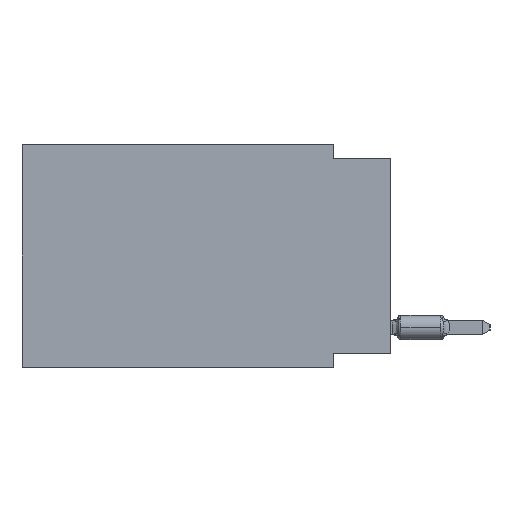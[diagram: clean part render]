
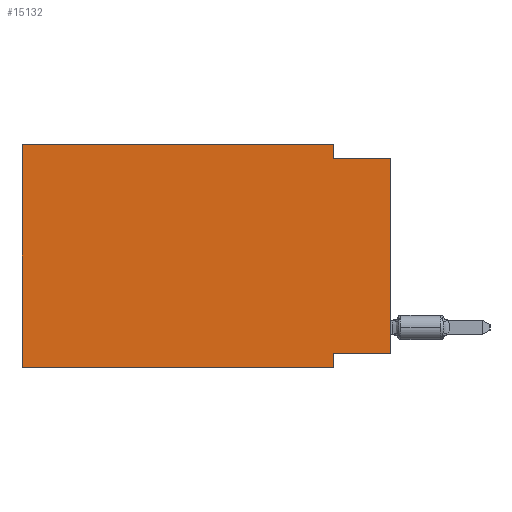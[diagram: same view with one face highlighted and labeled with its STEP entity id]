
A CAD part, left-side view. The second image highlights one B-rep face of the part: STEP entity #15132.
In plain terms, the highlighted planar face has unit normal (-1, 0, 0).
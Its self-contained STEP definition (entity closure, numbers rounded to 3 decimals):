
#46 = EDGE_CURVE ( 'NONE', #6103, #14184, #15102, .T. ) ;
#79 = CARTESIAN_POINT ( 'NONE',  ( 0., 16.383, -9.906 ) ) ;
#693 = ORIENTED_EDGE ( 'NONE', *, *, #7717, .T. ) ;
#972 = PLANE ( 'NONE',  #1155 ) ;
#1155 = AXIS2_PLACEMENT_3D ( 'NONE', #4593, #9602, #20739 ) ;
#1368 = EDGE_CURVE ( 'NONE', #10197, #13749, #8727, .T. ) ;
#1797 = ORIENTED_EDGE ( 'NONE', *, *, #46, .F. ) ;
#1824 = VECTOR ( 'NONE', #12740, 1000. ) ;
#1884 = CARTESIAN_POINT ( 'NONE',  ( 0., 2.54, 0. ) ) ;
#2053 = ORIENTED_EDGE ( 'NONE', *, *, #5603, .F. ) ;
#2114 = CARTESIAN_POINT ( 'NONE',  ( 0., 0., 0. ) ) ;
#2414 = VECTOR ( 'NONE', #20192, 1000. ) ;
#2853 = LINE ( 'NONE', #16040, #5142 ) ;
#2958 = CARTESIAN_POINT ( 'NONE',  ( 0., 2.54, -9.906 ) ) ;
#4232 = VECTOR ( 'NONE', #5402, 1000. ) ;
#4593 = CARTESIAN_POINT ( 'NONE',  ( 0., 16.383, 0. ) ) ;
#5037 = ORIENTED_EDGE ( 'NONE', *, *, #10943, .F. ) ;
#5142 = VECTOR ( 'NONE', #7863, 1000. ) ;
#5294 = ORIENTED_EDGE ( 'NONE', *, *, #17485, .F. ) ;
#5402 = DIRECTION ( 'NONE',  ( 0., 0., 1. ) ) ;
#5511 = LINE ( 'NONE', #2114, #4232 ) ;
#5603 = EDGE_CURVE ( 'NONE', #13749, #9847, #2853, .T. ) ;
#5905 = DIRECTION ( 'NONE',  ( 0., 0., -1. ) ) ;
#6055 = VERTEX_POINT ( 'NONE', #1884 ) ;
#6086 = LINE ( 'NONE', #12584, #6433 ) ;
#6103 = VERTEX_POINT ( 'NONE', #79 ) ;
#6238 = CARTESIAN_POINT ( 'NONE',  ( 0., 0., -0.635 ) ) ;
#6433 = VECTOR ( 'NONE', #17788, 1000. ) ;
#6855 = ORIENTED_EDGE ( 'NONE', *, *, #1368, .F. ) ;
#7028 = CARTESIAN_POINT ( 'NONE',  ( 0., 16.383, 0. ) ) ;
#7201 = CARTESIAN_POINT ( 'NONE',  ( 0., 2.54, 0. ) ) ;
#7248 = VECTOR ( 'NONE', #5905, 1000. ) ;
#7442 = ORIENTED_EDGE ( 'NONE', *, *, #8928, .F. ) ;
#7717 = EDGE_CURVE ( 'NONE', #10197, #11897, #5511, .T. ) ;
#7863 = DIRECTION ( 'NONE',  ( 0., 0., -1. ) ) ;
#7889 = LINE ( 'NONE', #19252, #13602 ) ;
#8727 = LINE ( 'NONE', #15091, #2414 ) ;
#8928 = EDGE_CURVE ( 'NONE', #6055, #10804, #17160, .T. ) ;
#9602 = DIRECTION ( 'NONE',  ( 1., 0., 0. ) ) ;
#9763 = LINE ( 'NONE', #6238, #1824 ) ;
#9847 = VERTEX_POINT ( 'NONE', #2958 ) ;
#10197 = VERTEX_POINT ( 'NONE', #11917 ) ;
#10804 = VERTEX_POINT ( 'NONE', #18928 ) ;
#10943 = EDGE_CURVE ( 'NONE', #14184, #6055, #7889, .T. ) ;
#11186 = FACE_OUTER_BOUND ( 'NONE', #15226, .T. ) ;
#11897 = VERTEX_POINT ( 'NONE', #20745 ) ;
#11917 = CARTESIAN_POINT ( 'NONE',  ( 0., 0., -9.271 ) ) ;
#12584 = CARTESIAN_POINT ( 'NONE',  ( 0., 16.383, -9.906 ) ) ;
#12740 = DIRECTION ( 'NONE',  ( 0., -1., 0. ) ) ;
#13602 = VECTOR ( 'NONE', #16068, 1000. ) ;
#13634 = EDGE_CURVE ( 'NONE', #6103, #9847, #6086, .T. ) ;
#13749 = VERTEX_POINT ( 'NONE', #17999 ) ;
#14184 = VERTEX_POINT ( 'NONE', #16994 ) ;
#15091 = CARTESIAN_POINT ( 'NONE',  ( 0., 0., -9.271 ) ) ;
#15102 = LINE ( 'NONE', #7028, #17742 ) ;
#15132 = ADVANCED_FACE ( 'NONE', ( #11186 ), #972, .F. ) ;
#15226 = EDGE_LOOP ( 'NONE', ( #693, #5294, #7442, #5037, #1797, #20839, #2053, #6855 ) ) ;
#15297 = DIRECTION ( 'NONE',  ( 0., 0., 1. ) ) ;
#16040 = CARTESIAN_POINT ( 'NONE',  ( 0., 2.54, -9.906 ) ) ;
#16068 = DIRECTION ( 'NONE',  ( 0., -1., 0. ) ) ;
#16994 = CARTESIAN_POINT ( 'NONE',  ( 0., 16.383, 0. ) ) ;
#17160 = LINE ( 'NONE', #7201, #7248 ) ;
#17485 = EDGE_CURVE ( 'NONE', #10804, #11897, #9763, .T. ) ;
#17742 = VECTOR ( 'NONE', #15297, 1000. ) ;
#17788 = DIRECTION ( 'NONE',  ( 0., -1., 0. ) ) ;
#17999 = CARTESIAN_POINT ( 'NONE',  ( 0., 2.54, -9.271 ) ) ;
#18928 = CARTESIAN_POINT ( 'NONE',  ( 0., 2.54, -0.635 ) ) ;
#19252 = CARTESIAN_POINT ( 'NONE',  ( 0., 16.383, 0. ) ) ;
#20192 = DIRECTION ( 'NONE',  ( 0., 1., 0. ) ) ;
#20739 = DIRECTION ( 'NONE',  ( 0., 0., -1. ) ) ;
#20745 = CARTESIAN_POINT ( 'NONE',  ( 0., 0., -0.635 ) ) ;
#20839 = ORIENTED_EDGE ( 'NONE', *, *, #13634, .T. ) ;
